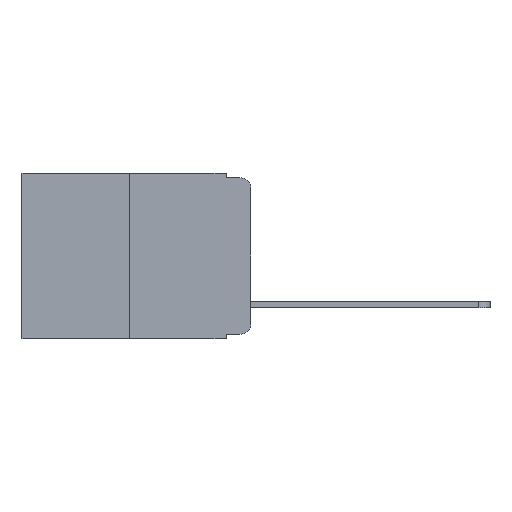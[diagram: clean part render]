
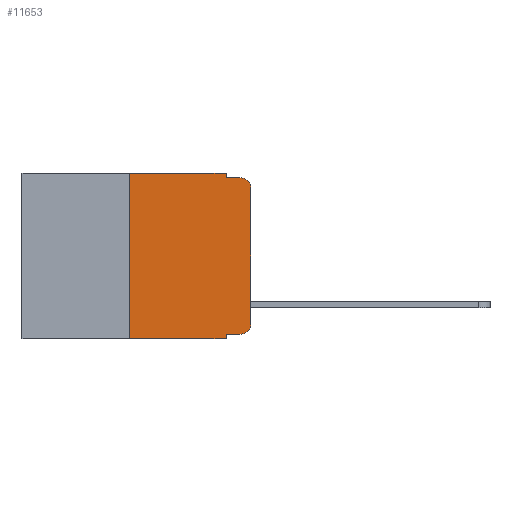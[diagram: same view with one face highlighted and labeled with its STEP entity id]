
A CAD part, left-side view. The second image highlights one B-rep face of the part: STEP entity #11653.
In plain terms, the highlighted planar face has unit normal (-1, 0, 0).
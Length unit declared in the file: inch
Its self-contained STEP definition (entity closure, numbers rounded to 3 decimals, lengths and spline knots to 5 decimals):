
#116 = ORIENTED_EDGE ( 'NONE', *, *, #9070, .T. ) ;
#133 = ORIENTED_EDGE ( 'NONE', *, *, #8422, .F. ) ;
#222 = VECTOR ( 'NONE', #1309, 39.37008 ) ;
#266 = ORIENTED_EDGE ( 'NONE', *, *, #8401, .T. ) ;
#354 = VERTEX_POINT ( 'NONE', #11511 ) ;
#410 = DIRECTION ( 'NONE',  ( -1., 0., 0. ) ) ;
#457 = DIRECTION ( 'NONE',  ( 0., 0., -1. ) ) ;
#477 = AXIS2_PLACEMENT_3D ( 'NONE', #6850, #410, #3227 ) ;
#531 = ORIENTED_EDGE ( 'NONE', *, *, #8421, .T. ) ;
#594 = VERTEX_POINT ( 'NONE', #10762 ) ;
#640 = CARTESIAN_POINT ( 'NONE',  ( 0., 0.051, 0. ) ) ;
#808 = CARTESIAN_POINT ( 'NONE',  ( 0., 0., 0. ) ) ;
#884 = AXIS2_PLACEMENT_3D ( 'NONE', #11386, #11362, #5411 ) ;
#961 = VERTEX_POINT ( 'NONE', #3301 ) ;
#1309 = DIRECTION ( 'NONE',  ( 0., -1., 0. ) ) ;
#1352 = VERTEX_POINT ( 'NONE', #10873 ) ;
#1550 = DIRECTION ( 'NONE',  ( 1., 0., 0. ) ) ;
#2128 = FACE_OUTER_BOUND ( 'NONE', #2162, .T. ) ;
#2162 = EDGE_LOOP ( 'NONE', ( #5195, #5225, #5335, #5349, #5429, #6034, #116, #133, #266, #531 ) ) ;
#2196 = VERTEX_POINT ( 'NONE', #11149 ) ;
#2303 = CARTESIAN_POINT ( 'NONE',  ( 0., 0.473, -0.343 ) ) ;
#2401 = LINE ( 'NONE', #2303, #9692 ) ;
#2895 = DIRECTION ( 'NONE',  ( 0., -1., 0. ) ) ;
#3119 = LINE ( 'NONE', #3184, #222 ) ;
#3184 = CARTESIAN_POINT ( 'NONE',  ( 0., 0.051, -0.333 ) ) ;
#3227 = DIRECTION ( 'NONE',  ( 0., 0., -1. ) ) ;
#3301 = CARTESIAN_POINT ( 'NONE',  ( 0., 0., -0.03 ) ) ;
#3304 = VERTEX_POINT ( 'NONE', #6228 ) ;
#3588 = VERTEX_POINT ( 'NONE', #4902 ) ;
#4754 = CARTESIAN_POINT ( 'NONE',  ( 0., 0.051, 0. ) ) ;
#4902 = CARTESIAN_POINT ( 'NONE',  ( 0., 0., -0.313 ) ) ;
#4977 = LINE ( 'NONE', #7769, #11559 ) ;
#5195 = ORIENTED_EDGE ( 'NONE', *, *, #8688, .T. ) ;
#5225 = ORIENTED_EDGE ( 'NONE', *, *, #8556, .T. ) ;
#5302 = VERTEX_POINT ( 'NONE', #6887 ) ;
#5335 = ORIENTED_EDGE ( 'NONE', *, *, #8619, .F. ) ;
#5349 = ORIENTED_EDGE ( 'NONE', *, *, #8457, .F. ) ;
#5411 = DIRECTION ( 'NONE',  ( 0., 0., -1. ) ) ;
#5429 = ORIENTED_EDGE ( 'NONE', *, *, #9594, .F. ) ;
#5699 = AXIS2_PLACEMENT_3D ( 'NONE', #7618, #1550, #8521 ) ;
#5714 = CIRCLE ( 'NONE', #477, 0.02 ) ;
#6013 = VECTOR ( 'NONE', #11071, 39.37008 ) ;
#6034 = ORIENTED_EDGE ( 'NONE', *, *, #8539, .F. ) ;
#6062 = DIRECTION ( 'NONE',  ( 0., -1., 0. ) ) ;
#6153 = LINE ( 'NONE', #808, #10439 ) ;
#6228 = CARTESIAN_POINT ( 'NONE',  ( 0., 0.051, -0.333 ) ) ;
#6561 = CARTESIAN_POINT ( 'NONE',  ( 0., 0.473, 0. ) ) ;
#6569 = VERTEX_POINT ( 'NONE', #640 ) ;
#6750 = VERTEX_POINT ( 'NONE', #7042 ) ;
#6850 = CARTESIAN_POINT ( 'NONE',  ( 0., 0.02, -0.03 ) ) ;
#6880 = CARTESIAN_POINT ( 'NONE',  ( 0., 0.25, 0. ) ) ;
#6887 = CARTESIAN_POINT ( 'NONE',  ( 0., 0.25, -0.343 ) ) ;
#7042 = CARTESIAN_POINT ( 'NONE',  ( 0., 0.25, 0. ) ) ;
#7538 = LINE ( 'NONE', #7687, #9111 ) ;
#7618 = CARTESIAN_POINT ( 'NONE',  ( 0., 0.473, 0. ) ) ;
#7687 = CARTESIAN_POINT ( 'NONE',  ( 0., 0.051, -0.01 ) ) ;
#7769 = CARTESIAN_POINT ( 'NONE',  ( 0., 0.051, 0. ) ) ;
#8335 = LINE ( 'NONE', #6561, #12310 ) ;
#8401 = EDGE_CURVE ( 'NONE', #3304, #1352, #3119, .T. ) ;
#8421 = EDGE_CURVE ( 'NONE', #1352, #3588, #9715, .T. ) ;
#8422 = EDGE_CURVE ( 'NONE', #3304, #2196, #4977, .T. ) ;
#8457 = EDGE_CURVE ( 'NONE', #6569, #594, #9229, .T. ) ;
#8479 = PLANE ( 'NONE',  #5699 ) ;
#8521 = DIRECTION ( 'NONE',  ( 0., 0., -1. ) ) ;
#8539 = EDGE_CURVE ( 'NONE', #5302, #6750, #10829, .T. ) ;
#8556 = EDGE_CURVE ( 'NONE', #961, #354, #5714, .T. ) ;
#8619 = EDGE_CURVE ( 'NONE', #594, #354, #7538, .T. ) ;
#8688 = EDGE_CURVE ( 'NONE', #3588, #961, #6153, .T. ) ;
#9070 = EDGE_CURVE ( 'NONE', #5302, #2196, #2401, .T. ) ;
#9111 = VECTOR ( 'NONE', #2895, 39.37008 ) ;
#9229 = LINE ( 'NONE', #4754, #11300 ) ;
#9577 = DIRECTION ( 'NONE',  ( 0., 0., 1. ) ) ;
#9594 = EDGE_CURVE ( 'NONE', #6750, #6569, #8335, .T. ) ;
#9609 = DIRECTION ( 'NONE',  ( 0., 0., -1. ) ) ;
#9692 = VECTOR ( 'NONE', #6062, 39.37008 ) ;
#9715 = CIRCLE ( 'NONE', #884, 0.02 ) ;
#10439 = VECTOR ( 'NONE', #9577, 39.37008 ) ;
#10762 = CARTESIAN_POINT ( 'NONE',  ( 0., 0.051, -0.01 ) ) ;
#10829 = LINE ( 'NONE', #6880, #6013 ) ;
#10873 = CARTESIAN_POINT ( 'NONE',  ( 0., 0.02, -0.333 ) ) ;
#11071 = DIRECTION ( 'NONE',  ( 0., 0., 1. ) ) ;
#11149 = CARTESIAN_POINT ( 'NONE',  ( 0., 0.051, -0.343 ) ) ;
#11300 = VECTOR ( 'NONE', #9609, 39.37008 ) ;
#11362 = DIRECTION ( 'NONE',  ( -1., 0., 0. ) ) ;
#11386 = CARTESIAN_POINT ( 'NONE',  ( 0., 0.02, -0.313 ) ) ;
#11511 = CARTESIAN_POINT ( 'NONE',  ( 0., 0.02, -0.01 ) ) ;
#11559 = VECTOR ( 'NONE', #457, 39.37008 ) ;
#11653 = ADVANCED_FACE ( 'NONE', ( #2128 ), #8479, .F. ) ;
#11838 = DIRECTION ( 'NONE',  ( 0., -1., 0. ) ) ;
#12310 = VECTOR ( 'NONE', #11838, 39.37008 ) ;
